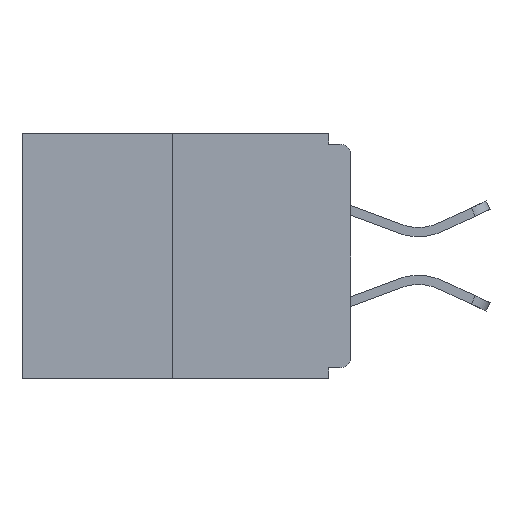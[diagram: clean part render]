
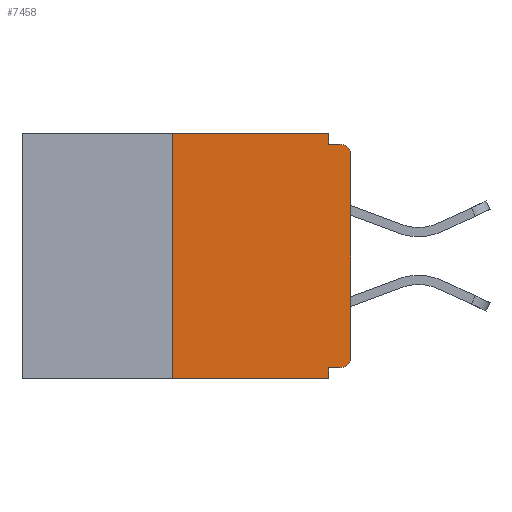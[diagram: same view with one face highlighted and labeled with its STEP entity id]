
A CAD part, left-side view. The second image highlights one B-rep face of the part: STEP entity #7458.
In plain terms, the highlighted planar face has unit normal (-1, 0, 0).
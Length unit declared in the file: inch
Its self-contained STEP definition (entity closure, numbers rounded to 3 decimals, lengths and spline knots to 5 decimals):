
#668 = DIRECTION ( 'NONE',  ( 0., 1., 0. ) ) ;
#955 = LINE ( 'NONE', #10110, #7061 ) ;
#970 = CARTESIAN_POINT ( 'NONE',  ( 0., 0.015, -0.313 ) ) ;
#1336 = VERTEX_POINT ( 'NONE', #11436 ) ;
#1518 = VERTEX_POINT ( 'NONE', #2651 ) ;
#1689 = CARTESIAN_POINT ( 'NONE',  ( 0., 0., -0.313 ) ) ;
#1735 = EDGE_CURVE ( 'NONE', #25077, #1336, #8278, .T. ) ;
#1771 = VERTEX_POINT ( 'NONE', #17471 ) ;
#2113 = EDGE_LOOP ( 'NONE', ( #22552, #14678, #15973, #6332, #26020, #21744, #3488, #14871, #15650, #12026 ) ) ;
#2241 = CARTESIAN_POINT ( 'NONE',  ( 0., 0.25, -0.343 ) ) ;
#2447 = CARTESIAN_POINT ( 'NONE',  ( 0., 0., -0.03 ) ) ;
#2651 = CARTESIAN_POINT ( 'NONE',  ( 0., 0.031, -0.015 ) ) ;
#2920 = AXIS2_PLACEMENT_3D ( 'NONE', #24342, #14236, #6244 ) ;
#3034 = DIRECTION ( 'NONE',  ( 0., 0., -1. ) ) ;
#3372 = LINE ( 'NONE', #4401, #21868 ) ;
#3488 = ORIENTED_EDGE ( 'NONE', *, *, #8306, .T. ) ;
#3826 = AXIS2_PLACEMENT_3D ( 'NONE', #26080, #3930, #17851 ) ;
#3930 = DIRECTION ( 'NONE',  ( -1., 0., 0. ) ) ;
#3935 = VERTEX_POINT ( 'NONE', #5493 ) ;
#4401 = CARTESIAN_POINT ( 'NONE',  ( 0., 0.46, -0.343 ) ) ;
#4593 = DIRECTION ( 'NONE',  ( 0., -1., 0. ) ) ;
#4787 = DIRECTION ( 'NONE',  ( 0., 0., -1. ) ) ;
#5493 = CARTESIAN_POINT ( 'NONE',  ( 0., 0.031, 0. ) ) ;
#5670 = VECTOR ( 'NONE', #668, 39.37008 ) ;
#5687 = EDGE_CURVE ( 'NONE', #14907, #15780, #12351, .T. ) ;
#6244 = DIRECTION ( 'NONE',  ( 0., 0., -1. ) ) ;
#6332 = ORIENTED_EDGE ( 'NONE', *, *, #18967, .F. ) ;
#7061 = VECTOR ( 'NONE', #12059, 39.37008 ) ;
#7175 = CARTESIAN_POINT ( 'NONE',  ( 0., 0.031, 0. ) ) ;
#7458 = ADVANCED_FACE ( 'NONE', ( #16718 ), #10248, .F. ) ;
#7895 = LINE ( 'NONE', #7175, #24162 ) ;
#8278 = LINE ( 'NONE', #15403, #16551 ) ;
#8306 = EDGE_CURVE ( 'NONE', #15012, #20765, #21446, .T. ) ;
#9011 = CARTESIAN_POINT ( 'NONE',  ( 0., 0.015, -0.328 ) ) ;
#9447 = CARTESIAN_POINT ( 'NONE',  ( 0., 0., 0. ) ) ;
#9641 = LINE ( 'NONE', #12701, #12502 ) ;
#10110 = CARTESIAN_POINT ( 'NONE',  ( 0., 0.46, 0. ) ) ;
#10248 = PLANE ( 'NONE',  #2920 ) ;
#10394 = DIRECTION ( 'NONE',  ( 0., -1., 0. ) ) ;
#10686 = CARTESIAN_POINT ( 'NONE',  ( 0., 0., -0.328 ) ) ;
#11057 = CIRCLE ( 'NONE', #3826, 0.015 ) ;
#11436 = CARTESIAN_POINT ( 'NONE',  ( 0., 0.25, 0. ) ) ;
#12026 = ORIENTED_EDGE ( 'NONE', *, *, #15859, .F. ) ;
#12059 = DIRECTION ( 'NONE',  ( 0., -1., 0. ) ) ;
#12209 = VECTOR ( 'NONE', #4787, 39.37008 ) ;
#12351 = LINE ( 'NONE', #10686, #5670 ) ;
#12502 = VECTOR ( 'NONE', #4593, 39.37008 ) ;
#12701 = CARTESIAN_POINT ( 'NONE',  ( 0., 0., -0.015 ) ) ;
#14236 = DIRECTION ( 'NONE',  ( 1., 0., 0. ) ) ;
#14678 = ORIENTED_EDGE ( 'NONE', *, *, #1735, .F. ) ;
#14679 = EDGE_CURVE ( 'NONE', #1336, #3935, #955, .T. ) ;
#14871 = ORIENTED_EDGE ( 'NONE', *, *, #16067, .T. ) ;
#14872 = EDGE_CURVE ( 'NONE', #14907, #15012, #15339, .T. ) ;
#14907 = VERTEX_POINT ( 'NONE', #9011 ) ;
#15012 = VERTEX_POINT ( 'NONE', #1689 ) ;
#15267 = VERTEX_POINT ( 'NONE', #22662 ) ;
#15339 = CIRCLE ( 'NONE', #21664, 0.015 ) ;
#15403 = CARTESIAN_POINT ( 'NONE',  ( 0., 0.25, 0. ) ) ;
#15650 = ORIENTED_EDGE ( 'NONE', *, *, #24826, .F. ) ;
#15780 = VERTEX_POINT ( 'NONE', #19283 ) ;
#15859 = EDGE_CURVE ( 'NONE', #3935, #1518, #7895, .T. ) ;
#15973 = ORIENTED_EDGE ( 'NONE', *, *, #22587, .T. ) ;
#16067 = EDGE_CURVE ( 'NONE', #20765, #15267, #11057, .T. ) ;
#16551 = VECTOR ( 'NONE', #17562, 39.37008 ) ;
#16718 = FACE_OUTER_BOUND ( 'NONE', #2113, .T. ) ;
#17471 = CARTESIAN_POINT ( 'NONE',  ( 0., 0.031, -0.343 ) ) ;
#17562 = DIRECTION ( 'NONE',  ( 0., 0., 1. ) ) ;
#17685 = CARTESIAN_POINT ( 'NONE',  ( 0., 0.031, -0.343 ) ) ;
#17851 = DIRECTION ( 'NONE',  ( 0., 0., -1. ) ) ;
#18967 = EDGE_CURVE ( 'NONE', #15780, #1771, #24353, .T. ) ;
#19283 = CARTESIAN_POINT ( 'NONE',  ( 0., 0.031, -0.328 ) ) ;
#19545 = DIRECTION ( 'NONE',  ( 0., 0., -1. ) ) ;
#19624 = DIRECTION ( 'NONE',  ( 0., 0., 1. ) ) ;
#20508 = VECTOR ( 'NONE', #19624, 39.37008 ) ;
#20765 = VERTEX_POINT ( 'NONE', #2447 ) ;
#21446 = LINE ( 'NONE', #9447, #20508 ) ;
#21664 = AXIS2_PLACEMENT_3D ( 'NONE', #970, #23641, #19545 ) ;
#21744 = ORIENTED_EDGE ( 'NONE', *, *, #14872, .T. ) ;
#21868 = VECTOR ( 'NONE', #10394, 39.37008 ) ;
#22552 = ORIENTED_EDGE ( 'NONE', *, *, #14679, .F. ) ;
#22587 = EDGE_CURVE ( 'NONE', #25077, #1771, #3372, .T. ) ;
#22662 = CARTESIAN_POINT ( 'NONE',  ( 0., 0.015, -0.015 ) ) ;
#23641 = DIRECTION ( 'NONE',  ( -1., 0., 0. ) ) ;
#24162 = VECTOR ( 'NONE', #3034, 39.37008 ) ;
#24342 = CARTESIAN_POINT ( 'NONE',  ( 0., 0.46, 0. ) ) ;
#24353 = LINE ( 'NONE', #17685, #12209 ) ;
#24826 = EDGE_CURVE ( 'NONE', #1518, #15267, #9641, .T. ) ;
#25077 = VERTEX_POINT ( 'NONE', #2241 ) ;
#26020 = ORIENTED_EDGE ( 'NONE', *, *, #5687, .F. ) ;
#26080 = CARTESIAN_POINT ( 'NONE',  ( 0., 0.015, -0.03 ) ) ;
